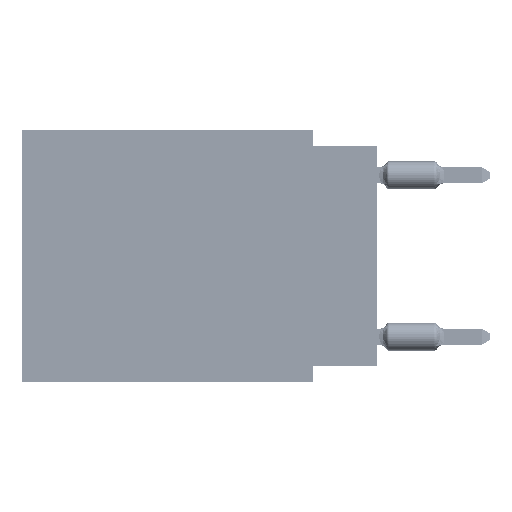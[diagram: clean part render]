
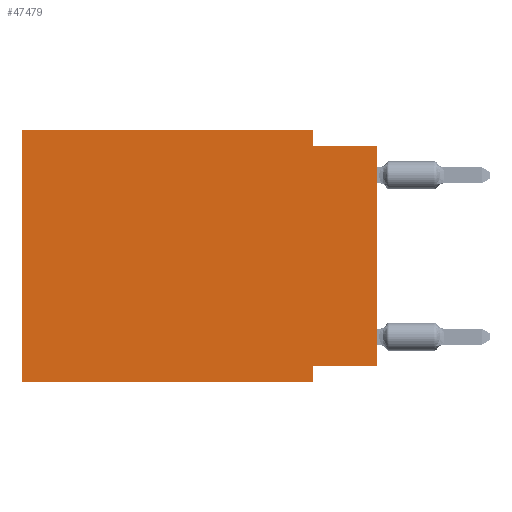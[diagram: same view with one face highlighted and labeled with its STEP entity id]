
A CAD part, left-side view. The second image highlights one B-rep face of the part: STEP entity #47479.
In plain terms, the highlighted planar face has unit normal (-1, 0, 0).
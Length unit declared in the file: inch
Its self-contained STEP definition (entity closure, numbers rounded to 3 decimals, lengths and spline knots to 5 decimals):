
#2193 = VERTEX_POINT ( 'NONE', #28437 ) ;
#3913 = EDGE_CURVE ( 'NONE', #36214, #64515, #43168, .T. ) ;
#5760 = LINE ( 'NONE', #42468, #15968 ) ;
#6208 = DIRECTION ( 'NONE',  ( 0., 0., -1. ) ) ;
#7460 = EDGE_CURVE ( 'NONE', #47178, #64515, #39267, .T. ) ;
#7959 = EDGE_CURVE ( 'NONE', #11045, #13479, #11203, .T. ) ;
#9258 = VECTOR ( 'NONE', #63265, 39.37008 ) ;
#10477 = DIRECTION ( 'NONE',  ( 0., 0., -1. ) ) ;
#10585 = DIRECTION ( 'NONE',  ( 0., 0., -1. ) ) ;
#11045 = VERTEX_POINT ( 'NONE', #71237 ) ;
#11203 = LINE ( 'NONE', #60662, #47211 ) ;
#11458 = VECTOR ( 'NONE', #14467, 39.37008 ) ;
#13479 = VERTEX_POINT ( 'NONE', #57189 ) ;
#13685 = ORIENTED_EDGE ( 'NONE', *, *, #31924, .F. ) ;
#14467 = DIRECTION ( 'NONE',  ( 0., 0., 1. ) ) ;
#15968 = VECTOR ( 'NONE', #10477, 39.37008 ) ;
#17812 = DIRECTION ( 'NONE',  ( 1., 0., 0. ) ) ;
#19280 = VECTOR ( 'NONE', #55290, 39.37008 ) ;
#19826 = ORIENTED_EDGE ( 'NONE', *, *, #7959, .T. ) ;
#20081 = CARTESIAN_POINT ( 'NONE',  ( 0., 0., -0.365 ) ) ;
#20148 = EDGE_CURVE ( 'NONE', #53654, #28869, #59504, .T. ) ;
#21470 = CARTESIAN_POINT ( 'NONE',  ( 0., 0.1, -0.39 ) ) ;
#23658 = ORIENTED_EDGE ( 'NONE', *, *, #55597, .F. ) ;
#24372 = CARTESIAN_POINT ( 'NONE',  ( 0., 0.55, 0. ) ) ;
#25787 = LINE ( 'NONE', #24372, #9258 ) ;
#26116 = EDGE_LOOP ( 'NONE', ( #53206, #56151, #27002, #68341, #13685, #19826, #23658, #69799 ) ) ;
#27002 = ORIENTED_EDGE ( 'NONE', *, *, #54364, .F. ) ;
#28437 = CARTESIAN_POINT ( 'NONE',  ( 0., 0.1, -0.365 ) ) ;
#28832 = VECTOR ( 'NONE', #10585, 39.37008 ) ;
#28869 = VERTEX_POINT ( 'NONE', #52780 ) ;
#30366 = AXIS2_PLACEMENT_3D ( 'NONE', #38914, #17812, #6208 ) ;
#31530 = CARTESIAN_POINT ( 'NONE',  ( 0., 0., 0. ) ) ;
#31836 = CARTESIAN_POINT ( 'NONE',  ( 0., 0.55, 0. ) ) ;
#31924 = EDGE_CURVE ( 'NONE', #11045, #53654, #25787, .T. ) ;
#33068 = CARTESIAN_POINT ( 'NONE',  ( 0., 0., -0.025 ) ) ;
#35138 = LINE ( 'NONE', #35494, #62149 ) ;
#35494 = CARTESIAN_POINT ( 'NONE',  ( 0., 0., -0.365 ) ) ;
#36214 = VERTEX_POINT ( 'NONE', #20081 ) ;
#38914 = CARTESIAN_POINT ( 'NONE',  ( 0., 0.55, 0. ) ) ;
#39267 = LINE ( 'NONE', #33068, #19280 ) ;
#39984 = FACE_OUTER_BOUND ( 'NONE', #26116, .T. ) ;
#41487 = CARTESIAN_POINT ( 'NONE',  ( 0., 0.1, -0.025 ) ) ;
#42468 = CARTESIAN_POINT ( 'NONE',  ( 0., 0.1, 0. ) ) ;
#42563 = LINE ( 'NONE', #21470, #28832 ) ;
#43168 = LINE ( 'NONE', #31530, #11458 ) ;
#47178 = VERTEX_POINT ( 'NONE', #41487 ) ;
#47211 = VECTOR ( 'NONE', #55201, 39.37008 ) ;
#47479 = ADVANCED_FACE ( 'NONE', ( #39984 ), #56025, .F. ) ;
#47940 = CARTESIAN_POINT ( 'NONE',  ( 0., 0., -0.025 ) ) ;
#52780 = CARTESIAN_POINT ( 'NONE',  ( 0., 0.1, 0. ) ) ;
#53206 = ORIENTED_EDGE ( 'NONE', *, *, #3913, .T. ) ;
#53654 = VERTEX_POINT ( 'NONE', #70476 ) ;
#54042 = DIRECTION ( 'NONE',  ( 0., -1., 0. ) ) ;
#54364 = EDGE_CURVE ( 'NONE', #28869, #47178, #5760, .T. ) ;
#55201 = DIRECTION ( 'NONE',  ( 0., -1., 0. ) ) ;
#55290 = DIRECTION ( 'NONE',  ( 0., -1., 0. ) ) ;
#55597 = EDGE_CURVE ( 'NONE', #2193, #13479, #42563, .T. ) ;
#56025 = PLANE ( 'NONE',  #30366 ) ;
#56151 = ORIENTED_EDGE ( 'NONE', *, *, #7460, .F. ) ;
#57189 = CARTESIAN_POINT ( 'NONE',  ( 0., 0.1, -0.39 ) ) ;
#57336 = DIRECTION ( 'NONE',  ( 0., 1., 0. ) ) ;
#59328 = VECTOR ( 'NONE', #54042, 39.37008 ) ;
#59504 = LINE ( 'NONE', #31836, #59328 ) ;
#60662 = CARTESIAN_POINT ( 'NONE',  ( 0., 0.55, -0.39 ) ) ;
#62149 = VECTOR ( 'NONE', #57336, 39.37008 ) ;
#63265 = DIRECTION ( 'NONE',  ( 0., 0., 1. ) ) ;
#64515 = VERTEX_POINT ( 'NONE', #47940 ) ;
#68341 = ORIENTED_EDGE ( 'NONE', *, *, #20148, .F. ) ;
#69799 = ORIENTED_EDGE ( 'NONE', *, *, #69878, .F. ) ;
#69878 = EDGE_CURVE ( 'NONE', #36214, #2193, #35138, .T. ) ;
#70476 = CARTESIAN_POINT ( 'NONE',  ( 0., 0.55, 0. ) ) ;
#71237 = CARTESIAN_POINT ( 'NONE',  ( 0., 0.55, -0.39 ) ) ;
